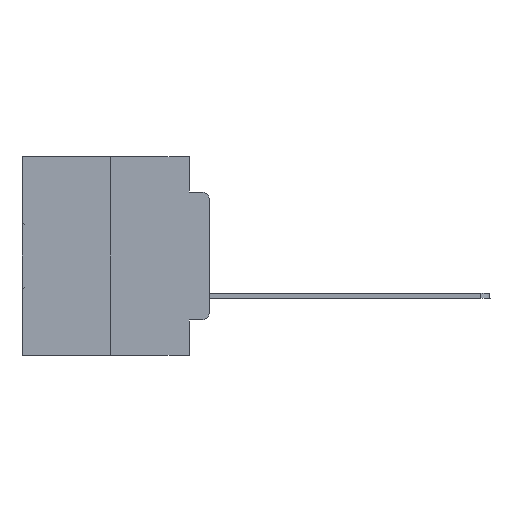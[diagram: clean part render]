
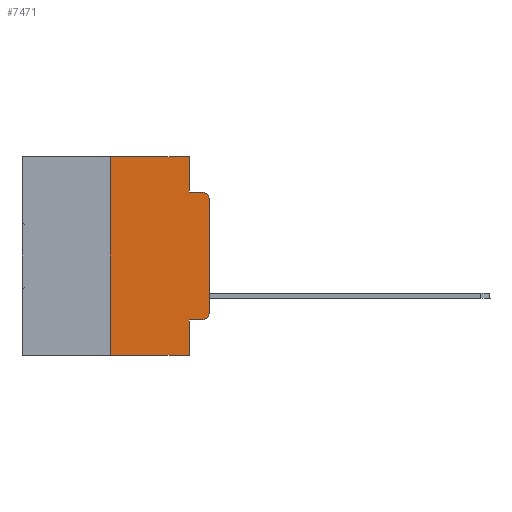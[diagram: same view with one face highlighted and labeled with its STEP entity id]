
A CAD part, left-side view. The second image highlights one B-rep face of the part: STEP entity #7471.
In plain terms, the highlighted planar face has unit normal (-1, 0, 0).
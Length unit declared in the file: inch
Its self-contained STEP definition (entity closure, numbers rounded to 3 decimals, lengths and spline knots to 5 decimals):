
#967 = CARTESIAN_POINT ( 'NONE',  ( 0., 0.25, 0. ) ) ;
#1927 = CARTESIAN_POINT ( 'NONE',  ( 0., 0.25, 0. ) ) ;
#2122 = CARTESIAN_POINT ( 'NONE',  ( 0., 0., -0.3915 ) ) ;
#2586 = AXIS2_PLACEMENT_3D ( 'NONE', #25985, #20812, #23713 ) ;
#2648 = EDGE_CURVE ( 'NONE', #5595, #28468, #9215, .T. ) ;
#3039 = PLANE ( 'NONE',  #2586 ) ;
#3242 = VERTEX_POINT ( 'NONE', #5309 ) ;
#3862 = ORIENTED_EDGE ( 'NONE', *, *, #25758, .T. ) ;
#3908 = ORIENTED_EDGE ( 'NONE', *, *, #9927, .F. ) ;
#4244 = CARTESIAN_POINT ( 'NONE',  ( 0., 0., 0. ) ) ;
#4713 = VERTEX_POINT ( 'NONE', #12780 ) ;
#4859 = ORIENTED_EDGE ( 'NONE', *, *, #21826, .T. ) ;
#5309 = CARTESIAN_POINT ( 'NONE',  ( 0., 0.02, -0.0885 ) ) ;
#5595 = VERTEX_POINT ( 'NONE', #2122 ) ;
#5968 = VERTEX_POINT ( 'NONE', #29186 ) ;
#6130 = DIRECTION ( 'NONE',  ( -1., 0., 0. ) ) ;
#6417 = DIRECTION ( 'NONE',  ( 0., -1., 0. ) ) ;
#6541 = CARTESIAN_POINT ( 'NONE',  ( 0., 0.02, -0.3915 ) ) ;
#7153 = LINE ( 'NONE', #24546, #30952 ) ;
#7289 = AXIS2_PLACEMENT_3D ( 'NONE', #6541, #24718, #22338 ) ;
#7416 = LINE ( 'NONE', #13673, #30809 ) ;
#7471 = ADVANCED_FACE ( 'NONE', ( #20972 ), #3039, .F. ) ;
#7762 = EDGE_LOOP ( 'NONE', ( #8988, #3862, #28940, #3908, #31149, #21502, #14357, #27293, #16331, #4859 ) ) ;
#8229 = LINE ( 'NONE', #30438, #21567 ) ;
#8772 = DIRECTION ( 'NONE',  ( 0., 0., 1. ) ) ;
#8786 = VERTEX_POINT ( 'NONE', #27532 ) ;
#8988 = ORIENTED_EDGE ( 'NONE', *, *, #2648, .T. ) ;
#9215 = LINE ( 'NONE', #4244, #16902 ) ;
#9927 = EDGE_CURVE ( 'NONE', #11981, #5968, #7153, .T. ) ;
#9968 = VECTOR ( 'NONE', #21067, 39.37008 ) ;
#10797 = EDGE_CURVE ( 'NONE', #20708, #8786, #8229, .T. ) ;
#11063 = DIRECTION ( 'NONE',  ( 0., -1., 0. ) ) ;
#11076 = DIRECTION ( 'NONE',  ( 0., -1., 0. ) ) ;
#11175 = CARTESIAN_POINT ( 'NONE',  ( 0., 0.473, -0.5 ) ) ;
#11462 = AXIS2_PLACEMENT_3D ( 'NONE', #27104, #6130, #14139 ) ;
#11981 = VERTEX_POINT ( 'NONE', #32857 ) ;
#12271 = VECTOR ( 'NONE', #11063, 39.37008 ) ;
#12780 = CARTESIAN_POINT ( 'NONE',  ( 0., 0.051, -0.5 ) ) ;
#13673 = CARTESIAN_POINT ( 'NONE',  ( 0., 0.051, -0.0885 ) ) ;
#14139 = DIRECTION ( 'NONE',  ( 0., 0., -1. ) ) ;
#14357 = ORIENTED_EDGE ( 'NONE', *, *, #15287, .T. ) ;
#14711 = EDGE_CURVE ( 'NONE', #29325, #25436, #31373, .T. ) ;
#14806 = LINE ( 'NONE', #15886, #9968 ) ;
#15206 = EDGE_CURVE ( 'NONE', #5968, #3242, #7416, .T. ) ;
#15214 = CARTESIAN_POINT ( 'NONE',  ( 0., 0.25, -0.5 ) ) ;
#15287 = EDGE_CURVE ( 'NONE', #29325, #4713, #32433, .T. ) ;
#15416 = CIRCLE ( 'NONE', #7289, 0.02 ) ;
#15886 = CARTESIAN_POINT ( 'NONE',  ( 0., 0.051, 0. ) ) ;
#16331 = ORIENTED_EDGE ( 'NONE', *, *, #10797, .T. ) ;
#16332 = CARTESIAN_POINT ( 'NONE',  ( 0., 0.473, 0. ) ) ;
#16902 = VECTOR ( 'NONE', #27485, 39.37008 ) ;
#17371 = DIRECTION ( 'NONE',  ( 0., -1., 0. ) ) ;
#18095 = LINE ( 'NONE', #16332, #26518 ) ;
#18945 = EDGE_CURVE ( 'NONE', #25436, #11981, #18095, .T. ) ;
#20708 = VERTEX_POINT ( 'NONE', #23760 ) ;
#20812 = DIRECTION ( 'NONE',  ( 1., 0., 0. ) ) ;
#20972 = FACE_OUTER_BOUND ( 'NONE', #7762, .T. ) ;
#21067 = DIRECTION ( 'NONE',  ( 0., 0., -1. ) ) ;
#21175 = CIRCLE ( 'NONE', #11462, 0.02 ) ;
#21502 = ORIENTED_EDGE ( 'NONE', *, *, #14711, .F. ) ;
#21567 = VECTOR ( 'NONE', #17371, 39.37008 ) ;
#21826 = EDGE_CURVE ( 'NONE', #8786, #5595, #15416, .T. ) ;
#22338 = DIRECTION ( 'NONE',  ( 0., 0., -1. ) ) ;
#23489 = CARTESIAN_POINT ( 'NONE',  ( 0., 0., -0.1085 ) ) ;
#23713 = DIRECTION ( 'NONE',  ( 0., 0., -1. ) ) ;
#23760 = CARTESIAN_POINT ( 'NONE',  ( 0., 0.051, -0.4115 ) ) ;
#24546 = CARTESIAN_POINT ( 'NONE',  ( 0., 0.051, 0. ) ) ;
#24718 = DIRECTION ( 'NONE',  ( -1., 0., 0. ) ) ;
#25436 = VERTEX_POINT ( 'NONE', #1927 ) ;
#25758 = EDGE_CURVE ( 'NONE', #28468, #3242, #21175, .T. ) ;
#25985 = CARTESIAN_POINT ( 'NONE',  ( 0., 0.473, 0. ) ) ;
#26518 = VECTOR ( 'NONE', #6417, 39.37008 ) ;
#26953 = VECTOR ( 'NONE', #8772, 39.37008 ) ;
#27104 = CARTESIAN_POINT ( 'NONE',  ( 0., 0.02, -0.1085 ) ) ;
#27293 = ORIENTED_EDGE ( 'NONE', *, *, #30079, .F. ) ;
#27485 = DIRECTION ( 'NONE',  ( 0., 0., 1. ) ) ;
#27532 = CARTESIAN_POINT ( 'NONE',  ( 0., 0.02, -0.4115 ) ) ;
#28468 = VERTEX_POINT ( 'NONE', #23489 ) ;
#28940 = ORIENTED_EDGE ( 'NONE', *, *, #15206, .F. ) ;
#29186 = CARTESIAN_POINT ( 'NONE',  ( 0., 0.051, -0.0885 ) ) ;
#29325 = VERTEX_POINT ( 'NONE', #15214 ) ;
#29714 = DIRECTION ( 'NONE',  ( 0., 0., -1. ) ) ;
#30079 = EDGE_CURVE ( 'NONE', #20708, #4713, #14806, .T. ) ;
#30438 = CARTESIAN_POINT ( 'NONE',  ( 0., 0.051, -0.4115 ) ) ;
#30809 = VECTOR ( 'NONE', #11076, 39.37008 ) ;
#30952 = VECTOR ( 'NONE', #29714, 39.37008 ) ;
#31149 = ORIENTED_EDGE ( 'NONE', *, *, #18945, .F. ) ;
#31373 = LINE ( 'NONE', #967, #26953 ) ;
#32433 = LINE ( 'NONE', #11175, #12271 ) ;
#32857 = CARTESIAN_POINT ( 'NONE',  ( 0., 0.051, 0. ) ) ;
